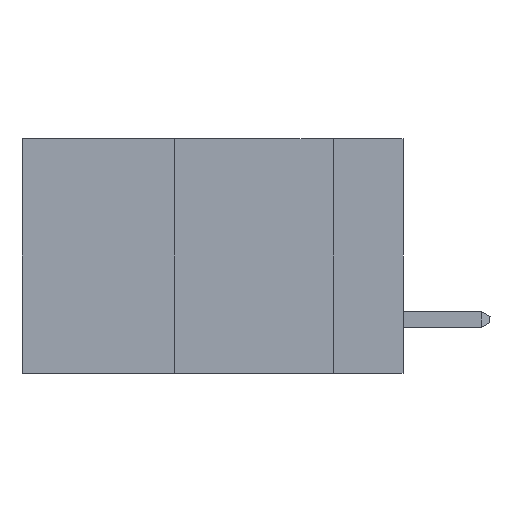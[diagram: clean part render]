
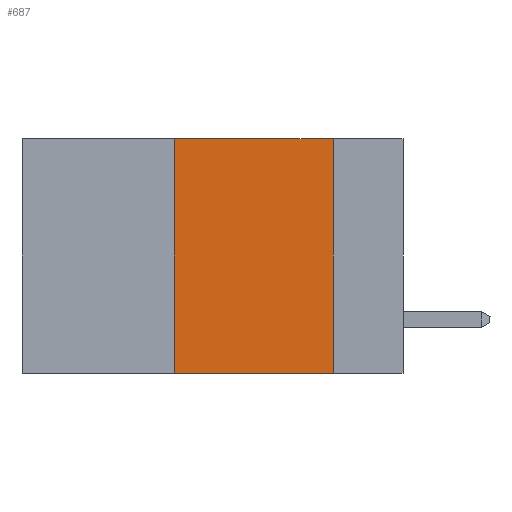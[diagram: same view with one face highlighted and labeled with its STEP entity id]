
A CAD part, left-side view. The second image highlights one B-rep face of the part: STEP entity #687.
In plain terms, the highlighted planar face has unit normal (-1, 0, 0).
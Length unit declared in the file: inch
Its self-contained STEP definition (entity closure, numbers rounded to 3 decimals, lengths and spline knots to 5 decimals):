
#412 = EDGE_CURVE ( 'NONE', #15537, #10958, #47179, .T. ) ;
#687 = ADVANCED_FACE ( 'NONE', ( #26693 ), #9047, .F. ) ;
#1110 = ORIENTED_EDGE ( 'NONE', *, *, #19572, .F. ) ;
#1736 = CARTESIAN_POINT ( 'NONE',  ( 0., 0.6, 0. ) ) ;
#3730 = VECTOR ( 'NONE', #13098, 39.37008 ) ;
#3928 = CARTESIAN_POINT ( 'NONE',  ( 0., 0.36, 0. ) ) ;
#8331 = VECTOR ( 'NONE', #43526, 39.37008 ) ;
#9047 = PLANE ( 'NONE',  #39758 ) ;
#10958 = VERTEX_POINT ( 'NONE', #44674 ) ;
#11480 = LINE ( 'NONE', #3928, #33753 ) ;
#13098 = DIRECTION ( 'NONE',  ( 0., -1., 0. ) ) ;
#13721 = LINE ( 'NONE', #28623, #8331 ) ;
#15537 = VERTEX_POINT ( 'NONE', #33847 ) ;
#19115 = CARTESIAN_POINT ( 'NONE',  ( 0., 0.36, -0.37 ) ) ;
#19572 = EDGE_CURVE ( 'NONE', #10958, #38390, #13721, .T. ) ;
#20199 = LINE ( 'NONE', #38999, #3730 ) ;
#25219 = DIRECTION ( 'NONE',  ( 0., -1., 0. ) ) ;
#26085 = ORIENTED_EDGE ( 'NONE', *, *, #412, .F. ) ;
#26693 = FACE_OUTER_BOUND ( 'NONE', #38587, .T. ) ;
#28154 = ORIENTED_EDGE ( 'NONE', *, *, #46503, .T. ) ;
#28623 = CARTESIAN_POINT ( 'NONE',  ( 0., 0.11, 0. ) ) ;
#31491 = CARTESIAN_POINT ( 'NONE',  ( 0., 0.11, -0.37 ) ) ;
#33578 = VERTEX_POINT ( 'NONE', #19115 ) ;
#33753 = VECTOR ( 'NONE', #44936, 39.37008 ) ;
#33847 = CARTESIAN_POINT ( 'NONE',  ( 0., 0.36, 0. ) ) ;
#33988 = EDGE_CURVE ( 'NONE', #33578, #15537, #11480, .T. ) ;
#36194 = CARTESIAN_POINT ( 'NONE',  ( 0., 0.6, 0. ) ) ;
#38390 = VERTEX_POINT ( 'NONE', #31491 ) ;
#38587 = EDGE_LOOP ( 'NONE', ( #1110, #26085, #48190, #28154 ) ) ;
#38839 = VECTOR ( 'NONE', #25219, 39.37008 ) ;
#38999 = CARTESIAN_POINT ( 'NONE',  ( 0., 0.6, -0.37 ) ) ;
#39758 = AXIS2_PLACEMENT_3D ( 'NONE', #1736, #46178, #41581 ) ;
#41581 = DIRECTION ( 'NONE',  ( 0., 0., -1. ) ) ;
#43526 = DIRECTION ( 'NONE',  ( 0., 0., -1. ) ) ;
#44674 = CARTESIAN_POINT ( 'NONE',  ( 0., 0.11, 0. ) ) ;
#44936 = DIRECTION ( 'NONE',  ( 0., 0., 1. ) ) ;
#46178 = DIRECTION ( 'NONE',  ( 1., 0., 0. ) ) ;
#46503 = EDGE_CURVE ( 'NONE', #33578, #38390, #20199, .T. ) ;
#47179 = LINE ( 'NONE', #36194, #38839 ) ;
#48190 = ORIENTED_EDGE ( 'NONE', *, *, #33988, .F. ) ;
